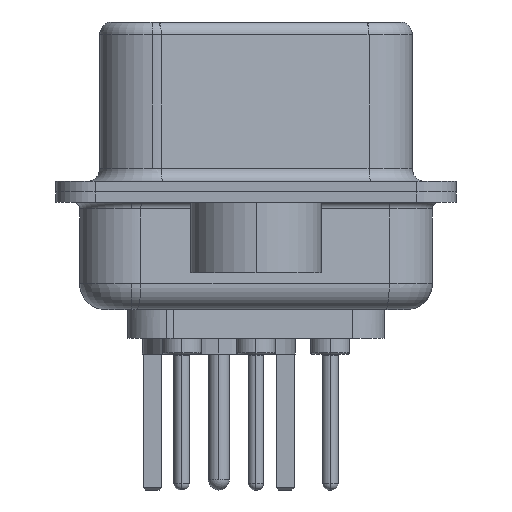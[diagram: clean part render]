
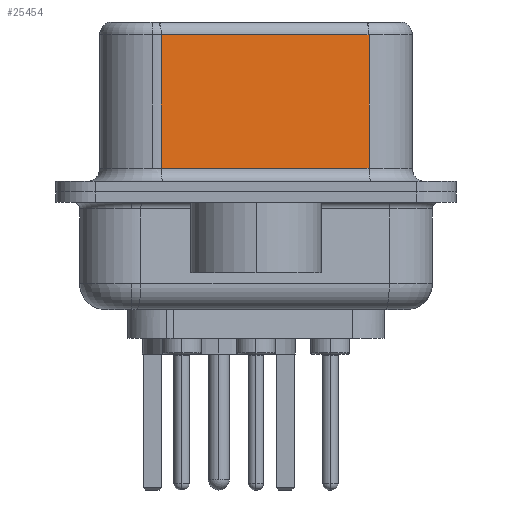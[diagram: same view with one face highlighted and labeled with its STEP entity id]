
A CAD part, left-side view. The second image highlights one B-rep face of the part: STEP entity #25454.
In plain terms, the highlighted planar face has unit normal (-0.985, -0.174, 0).
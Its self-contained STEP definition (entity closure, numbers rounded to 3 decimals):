
#3049 = VERTEX_POINT ( 'NONE', #28933 ) ;
#4490 = EDGE_CURVE ( 'NONE', #17360, #3049, #13246, .T. ) ;
#5496 = EDGE_CURVE ( 'NONE', #13270, #17360, #29902, .T. ) ;
#5634 = DIRECTION ( 'NONE',  ( 0., 0., -1. ) ) ;
#6107 = DIRECTION ( 'NONE',  ( 0., 0., -1. ) ) ;
#7498 = VECTOR ( 'NONE', #5634, 1000. ) ;
#9658 = PLANE ( 'NONE',  #24257 ) ;
#10860 = EDGE_CURVE ( 'NONE', #13270, #15097, #30806, .T. ) ;
#11787 = DIRECTION ( 'NONE',  ( -0.174, 0.985, 0. ) ) ;
#12001 = CARTESIAN_POINT ( 'NONE',  ( 3.73, 3.628, 6.02 ) ) ;
#12315 = CARTESIAN_POINT ( 'NONE',  ( 5.132, -4.322, 0.9 ) ) ;
#13246 = LINE ( 'NONE', #30227, #7498 ) ;
#13270 = VERTEX_POINT ( 'NONE', #22590 ) ;
#14196 = ORIENTED_EDGE ( 'NONE', *, *, #10860, .F. ) ;
#14348 = CARTESIAN_POINT ( 'NONE',  ( 5.132, -4.322, 6.52 ) ) ;
#15097 = VERTEX_POINT ( 'NONE', #16123 ) ;
#15991 = VECTOR ( 'NONE', #6107, 1000. ) ;
#16123 = CARTESIAN_POINT ( 'NONE',  ( 5.132, -4.322, 0.9 ) ) ;
#16517 = DIRECTION ( 'NONE',  ( 0.985, 0.174, 0. ) ) ;
#16666 = VECTOR ( 'NONE', #19878, 1000. ) ;
#17360 = VERTEX_POINT ( 'NONE', #12001 ) ;
#18518 = CARTESIAN_POINT ( 'NONE',  ( 5.132, -4.322, 6.52 ) ) ;
#19878 = DIRECTION ( 'NONE',  ( -0.174, 0.985, 0. ) ) ;
#22590 = CARTESIAN_POINT ( 'NONE',  ( 5.132, -4.322, 6.02 ) ) ;
#23243 = LINE ( 'NONE', #12315, #29086 ) ;
#23403 = ORIENTED_EDGE ( 'NONE', *, *, #5496, .T. ) ;
#24050 = FACE_OUTER_BOUND ( 'NONE', #24364, .T. ) ;
#24257 = AXIS2_PLACEMENT_3D ( 'NONE', #14348, #16517, #11787 ) ;
#24364 = EDGE_LOOP ( 'NONE', ( #14196, #23403, #31192, #28355 ) ) ;
#24589 = DIRECTION ( 'NONE',  ( 0.174, -0.985, 0. ) ) ;
#24680 = CARTESIAN_POINT ( 'NONE',  ( 5.132, -4.322, 6.02 ) ) ;
#25454 = ADVANCED_FACE ( 'NONE', ( #24050 ), #9658, .F. ) ;
#25574 = EDGE_CURVE ( 'NONE', #3049, #15097, #23243, .T. ) ;
#28355 = ORIENTED_EDGE ( 'NONE', *, *, #25574, .T. ) ;
#28933 = CARTESIAN_POINT ( 'NONE',  ( 3.73, 3.628, 0.9 ) ) ;
#29086 = VECTOR ( 'NONE', #24589, 1000. ) ;
#29902 = LINE ( 'NONE', #24680, #16666 ) ;
#30227 = CARTESIAN_POINT ( 'NONE',  ( 3.73, 3.628, 6.52 ) ) ;
#30806 = LINE ( 'NONE', #18518, #15991 ) ;
#31192 = ORIENTED_EDGE ( 'NONE', *, *, #4490, .T. ) ;
